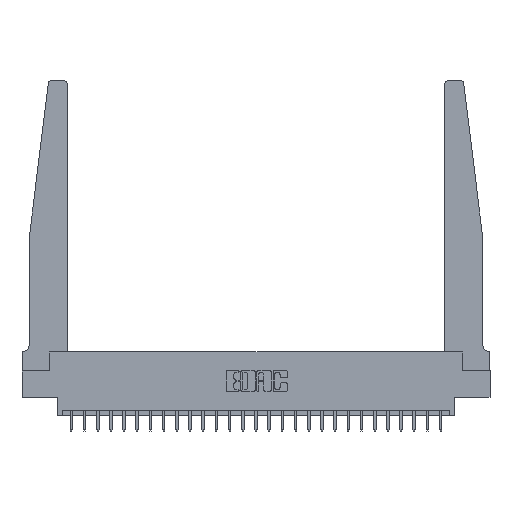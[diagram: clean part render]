
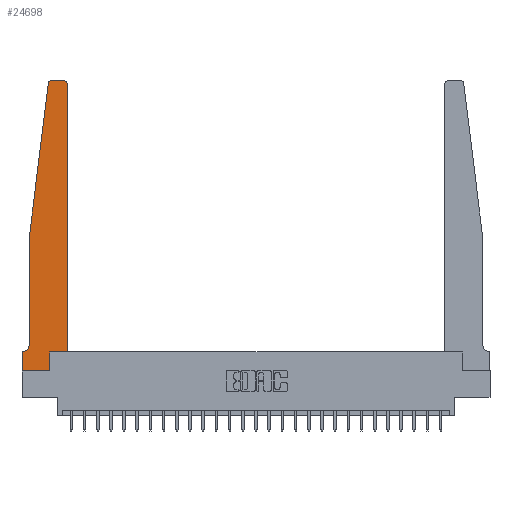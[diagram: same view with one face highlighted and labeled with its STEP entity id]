
A CAD part, top view. The second image highlights one B-rep face of the part: STEP entity #24698.
In plain terms, the highlighted planar face has unit normal (0, 0, 1).
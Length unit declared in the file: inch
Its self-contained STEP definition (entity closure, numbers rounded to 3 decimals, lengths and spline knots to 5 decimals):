
#11 = ORIENTED_EDGE ( 'NONE', *, *, #14042, .T. ) ;
#560 = ORIENTED_EDGE ( 'NONE', *, *, #13188, .T. ) ;
#691 = EDGE_CURVE ( 'NONE', #2700, #14562, #18083, .T. ) ;
#865 = DIRECTION ( 'NONE',  ( 1., 0., 0. ) ) ;
#953 = CARTESIAN_POINT ( 'NONE',  ( 0.425, 0.18, 0.37 ) ) ;
#1360 = CARTESIAN_POINT ( 'NONE',  ( 0.425, 0.18, 0.37 ) ) ;
#1605 = DIRECTION ( 'NONE',  ( -0.122, -0.992, 0. ) ) ;
#1885 = ORIENTED_EDGE ( 'NONE', *, *, #22488, .T. ) ;
#2270 = VECTOR ( 'NONE', #11987, 39.37008 ) ;
#2444 = VERTEX_POINT ( 'NONE', #16148 ) ;
#2506 = DIRECTION ( 'NONE',  ( 0., 0., 1. ) ) ;
#2700 = VERTEX_POINT ( 'NONE', #16891 ) ;
#3182 = ORIENTED_EDGE ( 'NONE', *, *, #691, .T. ) ;
#3445 = VECTOR ( 'NONE', #7008, 39.37008 ) ;
#3977 = DIRECTION ( 'NONE',  ( 0., 0., -1. ) ) ;
#4069 = LINE ( 'NONE', #953, #3445 ) ;
#4961 = LINE ( 'NONE', #9136, #25318 ) ;
#5143 = VERTEX_POINT ( 'NONE', #9696 ) ;
#5233 = EDGE_CURVE ( 'NONE', #11796, #20198, #17003, .T. ) ;
#5244 = CARTESIAN_POINT ( 'NONE',  ( 0.27653, 2.72, 0.37 ) ) ;
#5777 = CARTESIAN_POINT ( 'NONE',  ( 0., 0., 0.37 ) ) ;
#5849 = CARTESIAN_POINT ( 'NONE',  ( 0.065, 0.2375, 0.37 ) ) ;
#5850 = VERTEX_POINT ( 'NONE', #5849 ) ;
#6005 = CARTESIAN_POINT ( 'NONE',  ( 0.2605, 0.18, 0.37 ) ) ;
#6294 = CARTESIAN_POINT ( 'NONE',  ( 0.27653, 2.75, 0.37 ) ) ;
#6459 = CARTESIAN_POINT ( 'NONE',  ( 0., 0.1875, 0.37 ) ) ;
#6663 = CARTESIAN_POINT ( 'NONE',  ( 0., 0., 0.37 ) ) ;
#6825 = CARTESIAN_POINT ( 'NONE',  ( 0.425, 0.18, 0.37 ) ) ;
#6959 = VECTOR ( 'NONE', #15723, 39.37008 ) ;
#7008 = DIRECTION ( 'NONE',  ( 0., 1., 0. ) ) ;
#7265 = DIRECTION ( 'NONE',  ( 0., -1., 0. ) ) ;
#7267 = ORIENTED_EDGE ( 'NONE', *, *, #23930, .T. ) ;
#7276 = DIRECTION ( 'NONE',  ( 1., 0., 0. ) ) ;
#7342 = VERTEX_POINT ( 'NONE', #6663 ) ;
#7933 = VECTOR ( 'NONE', #7265, 39.37008 ) ;
#8669 = VERTEX_POINT ( 'NONE', #10495 ) ;
#9136 = CARTESIAN_POINT ( 'NONE',  ( 0., 0., 0.37 ) ) ;
#9511 = ORIENTED_EDGE ( 'NONE', *, *, #13340, .T. ) ;
#9696 = CARTESIAN_POINT ( 'NONE',  ( 0.065, 1.25, 0.37 ) ) ;
#9726 = EDGE_CURVE ( 'NONE', #14562, #7342, #12170, .T. ) ;
#9880 = AXIS2_PLACEMENT_3D ( 'NONE', #6459, #2506, #16371 ) ;
#10021 = CARTESIAN_POINT ( 'NONE',  ( 0.065, 0.1875, 0.37 ) ) ;
#10041 = DIRECTION ( 'NONE',  ( 0., 1., 0. ) ) ;
#10426 = PLANE ( 'NONE',  #9880 ) ;
#10465 = VERTEX_POINT ( 'NONE', #17762 ) ;
#10495 = CARTESIAN_POINT ( 'NONE',  ( 0.24675, 2.72367, 0.37 ) ) ;
#10577 = AXIS2_PLACEMENT_3D ( 'NONE', #5244, #19107, #7276 ) ;
#10982 = VECTOR ( 'NONE', #14760, 39.37008 ) ;
#11796 = VERTEX_POINT ( 'NONE', #12220 ) ;
#11837 = ORIENTED_EDGE ( 'NONE', *, *, #19344, .T. ) ;
#11987 = DIRECTION ( 'NONE',  ( -1., 0., 0. ) ) ;
#12087 = AXIS2_PLACEMENT_3D ( 'NONE', #24581, #12762, #865 ) ;
#12170 = LINE ( 'NONE', #5777, #6959 ) ;
#12220 = CARTESIAN_POINT ( 'NONE',  ( 0.2605, 0., 0.37 ) ) ;
#12649 = FACE_OUTER_BOUND ( 'NONE', #19037, .T. ) ;
#12762 = DIRECTION ( 'NONE',  ( 0., 0., 1. ) ) ;
#12840 = EDGE_CURVE ( 'NONE', #8669, #5143, #24880, .T. ) ;
#13188 = EDGE_CURVE ( 'NONE', #20198, #18884, #16235, .T. ) ;
#13191 = CARTESIAN_POINT ( 'NONE',  ( 0.065, 1.25, 0.37 ) ) ;
#13340 = EDGE_CURVE ( 'NONE', #5143, #5850, #13758, .T. ) ;
#13643 = DIRECTION ( 'NONE',  ( -1., 0., 0. ) ) ;
#13758 = LINE ( 'NONE', #13191, #7933 ) ;
#13785 = VECTOR ( 'NONE', #1605, 39.37008 ) ;
#14042 = EDGE_CURVE ( 'NONE', #19737, #8669, #15645, .T. ) ;
#14562 = VERTEX_POINT ( 'NONE', #14822 ) ;
#14760 = DIRECTION ( 'NONE',  ( 1., 0., 0. ) ) ;
#14822 = CARTESIAN_POINT ( 'NONE',  ( 0., 0.1875, 0.37 ) ) ;
#15488 = CARTESIAN_POINT ( 'NONE',  ( 0.065, 1.25, 0.37 ) ) ;
#15645 = CIRCLE ( 'NONE', #10577, 0.03 ) ;
#15723 = DIRECTION ( 'NONE',  ( 0., -1., 0. ) ) ;
#15841 = CARTESIAN_POINT ( 'NONE',  ( 0.015, 0.2375, 0.37 ) ) ;
#16148 = CARTESIAN_POINT ( 'NONE',  ( 0.395, 2.75, 0.37 ) ) ;
#16235 = LINE ( 'NONE', #6825, #10982 ) ;
#16371 = DIRECTION ( 'NONE',  ( 1., 0., 0. ) ) ;
#16500 = ORIENTED_EDGE ( 'NONE', *, *, #23128, .T. ) ;
#16891 = CARTESIAN_POINT ( 'NONE',  ( 0.015, 0.1875, 0.37 ) ) ;
#17003 = LINE ( 'NONE', #19899, #21075 ) ;
#17550 = ORIENTED_EDGE ( 'NONE', *, *, #9726, .T. ) ;
#17649 = CIRCLE ( 'NONE', #25503, 0.05 ) ;
#17762 = CARTESIAN_POINT ( 'NONE',  ( 0.425, 2.72, 0.37 ) ) ;
#17832 = DIRECTION ( 'NONE',  ( -1., 0., 0. ) ) ;
#18083 = LINE ( 'NONE', #10021, #2270 ) ;
#18884 = VERTEX_POINT ( 'NONE', #1360 ) ;
#19037 = EDGE_LOOP ( 'NONE', ( #7267, #11, #20689, #9511, #23089, #3182, #17550, #16500, #25202, #560, #1885, #11837 ) ) ;
#19107 = DIRECTION ( 'NONE',  ( 0., 0., 1. ) ) ;
#19185 = VECTOR ( 'NONE', #13643, 39.37008 ) ;
#19344 = EDGE_CURVE ( 'NONE', #10465, #2444, #24625, .T. ) ;
#19737 = VERTEX_POINT ( 'NONE', #6294 ) ;
#19800 = LINE ( 'NONE', #21563, #19185 ) ;
#19899 = CARTESIAN_POINT ( 'NONE',  ( 0.2605, 0.18, 0.37 ) ) ;
#20198 = VERTEX_POINT ( 'NONE', #6005 ) ;
#20689 = ORIENTED_EDGE ( 'NONE', *, *, #12840, .T. ) ;
#21075 = VECTOR ( 'NONE', #10041, 39.37008 ) ;
#21563 = CARTESIAN_POINT ( 'NONE',  ( 0.25, 2.75, 0.37 ) ) ;
#22488 = EDGE_CURVE ( 'NONE', #18884, #10465, #4069, .T. ) ;
#22942 = DIRECTION ( 'NONE',  ( 1., 0., 0. ) ) ;
#23089 = ORIENTED_EDGE ( 'NONE', *, *, #23307, .T. ) ;
#23128 = EDGE_CURVE ( 'NONE', #7342, #11796, #4961, .T. ) ;
#23307 = EDGE_CURVE ( 'NONE', #5850, #2700, #17649, .T. ) ;
#23930 = EDGE_CURVE ( 'NONE', #2444, #19737, #19800, .T. ) ;
#24581 = CARTESIAN_POINT ( 'NONE',  ( 0.395, 2.72, 0.37 ) ) ;
#24625 = CIRCLE ( 'NONE', #12087, 0.03 ) ;
#24698 = ADVANCED_FACE ( 'NONE', ( #12649 ), #10426, .T. ) ;
#24880 = LINE ( 'NONE', #15488, #13785 ) ;
#25202 = ORIENTED_EDGE ( 'NONE', *, *, #5233, .T. ) ;
#25318 = VECTOR ( 'NONE', #22942, 39.37008 ) ;
#25503 = AXIS2_PLACEMENT_3D ( 'NONE', #15841, #3977, #17832 ) ;
